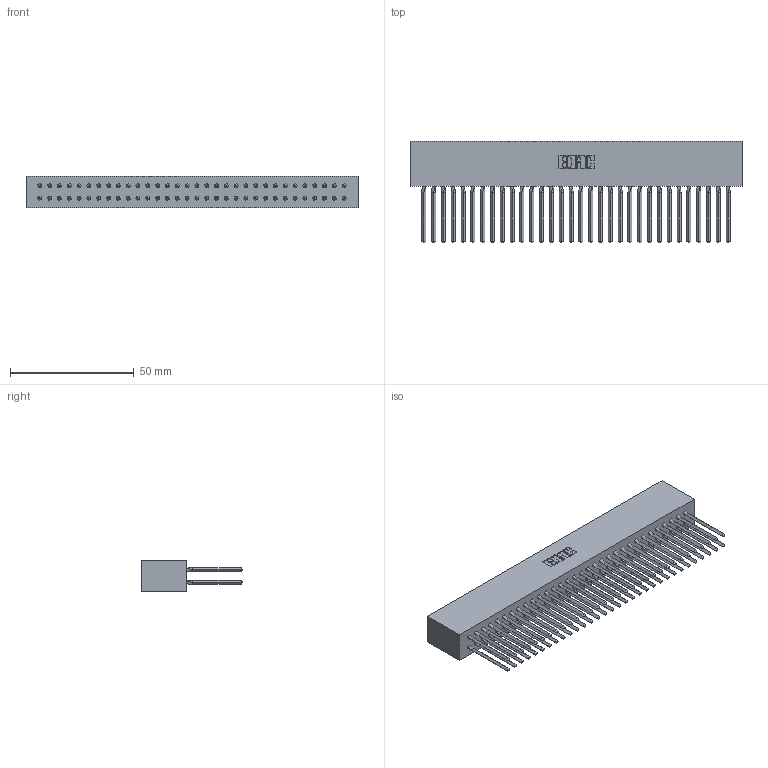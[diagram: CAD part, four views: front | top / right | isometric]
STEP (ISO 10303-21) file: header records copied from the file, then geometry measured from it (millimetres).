
FILE_DESCRIPTION (( 'STEP AP203' ), '1' );
FILE_NAME ('317-064-543-801.STEP', '2020-02-28T05:58:55', ( '' ), ( '' ), 'SwSTEP 2.0', 'SolidWorks 2016', '' );
FILE_SCHEMA (( 'CONFIG_CONTROL_DESIGN' ));
Length unit declared in the file: inch
Products named in the file (3): 317 Part_Lugless; 317-064-543-801; 317-290-001_543
Assembly tree (65 placements, depth 2):
  317-064-543-801
    317 Part_Lugless
    317-290-001_543  x64
Bounding box: 134.01 x 41.15 x 12.7 mm (x, y, z)
Volume: 24265.1 mm3; surface area: 36696 mm2
Topology: 65 solids, 65 shells, 5786 faces, 16047 edges, 10334 vertices
Faces by surface type: plane 4722, cylinder 808, bspline 256
Entity records: 47242 total; most frequent: CARTESIAN_POINT 8655, ORIENTED_EDGE 8154, DIRECTION 6795, EDGE_CURVE 4077, LINE 3829, VECTOR 3829, VERTEX_POINT 2711, AXIS2_PLACEMENT_3D 1483
